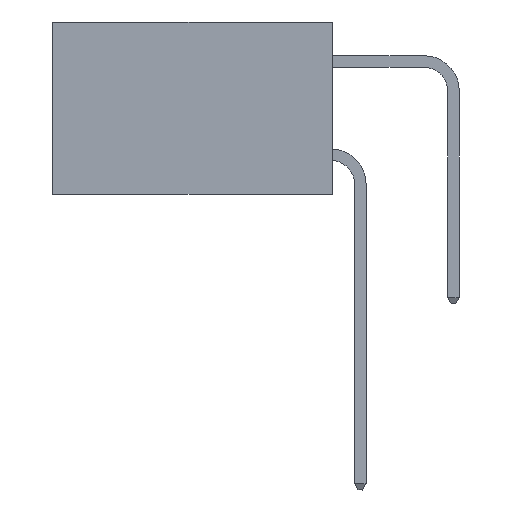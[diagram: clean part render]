
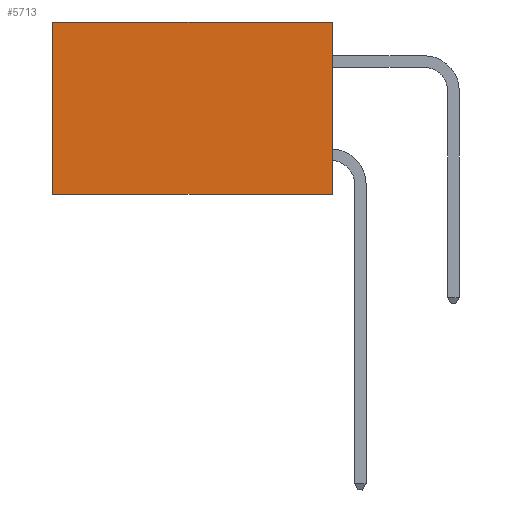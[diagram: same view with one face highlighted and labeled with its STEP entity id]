
A CAD part, left-side view. The second image highlights one B-rep face of the part: STEP entity #5713.
In plain terms, the highlighted planar face has unit normal (-1, 0, 0).
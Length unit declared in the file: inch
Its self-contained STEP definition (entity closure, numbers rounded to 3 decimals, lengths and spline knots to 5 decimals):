
#2286 = CARTESIAN_POINT ( 'NONE',  ( 0.298, 0., 0. ) ) ;
#3651 = ORIENTED_EDGE ( 'NONE', *, *, #4596, .T. ) ;
#4030 = VECTOR ( 'NONE', #24999, 39.37008 ) ;
#4124 = EDGE_CURVE ( 'NONE', #7701, #14958, #17705, .T. ) ;
#4596 = EDGE_CURVE ( 'NONE', #7062, #14991, #12025, .T. ) ;
#5713 = ADVANCED_FACE ( 'NONE', ( #29328 ), #16380, .F. ) ;
#6636 = ORIENTED_EDGE ( 'NONE', *, *, #4124, .F. ) ;
#7062 = VERTEX_POINT ( 'NONE', #23262 ) ;
#7609 = AXIS2_PLACEMENT_3D ( 'NONE', #8755, #13903, #31976 ) ;
#7701 = VERTEX_POINT ( 'NONE', #27364 ) ;
#8755 = CARTESIAN_POINT ( 'NONE',  ( 0.298, 0., 0. ) ) ;
#8858 = VECTOR ( 'NONE', #30581, 39.37008 ) ;
#10605 = CARTESIAN_POINT ( 'NONE',  ( 0.298, 0., -0.37 ) ) ;
#10717 = DIRECTION ( 'NONE',  ( 0., 1., 0. ) ) ;
#11938 = CARTESIAN_POINT ( 'NONE',  ( 0.298, 0.6, -0.37 ) ) ;
#12025 = LINE ( 'NONE', #2286, #8858 ) ;
#13350 = LINE ( 'NONE', #19286, #24247 ) ;
#13873 = ORIENTED_EDGE ( 'NONE', *, *, #21202, .F. ) ;
#13903 = DIRECTION ( 'NONE',  ( 1., 0., 0. ) ) ;
#14433 = CARTESIAN_POINT ( 'NONE',  ( 0.298, 0.6, 0. ) ) ;
#14958 = VERTEX_POINT ( 'NONE', #11938 ) ;
#14991 = VERTEX_POINT ( 'NONE', #16993 ) ;
#16380 = PLANE ( 'NONE',  #7609 ) ;
#16993 = CARTESIAN_POINT ( 'NONE',  ( 0.298, 0.6, 0. ) ) ;
#17705 = LINE ( 'NONE', #10605, #22547 ) ;
#19286 = CARTESIAN_POINT ( 'NONE',  ( 0.298, 0., 0. ) ) ;
#21202 = EDGE_CURVE ( 'NONE', #7062, #7701, #13350, .T. ) ;
#21790 = DIRECTION ( 'NONE',  ( 0., 0., -1. ) ) ;
#21914 = EDGE_CURVE ( 'NONE', #14991, #14958, #31548, .T. ) ;
#22331 = EDGE_LOOP ( 'NONE', ( #30204, #6636, #13873, #3651 ) ) ;
#22547 = VECTOR ( 'NONE', #10717, 39.37008 ) ;
#23262 = CARTESIAN_POINT ( 'NONE',  ( 0.298, 0., 0. ) ) ;
#24247 = VECTOR ( 'NONE', #21790, 39.37008 ) ;
#24999 = DIRECTION ( 'NONE',  ( 0., 0., -1. ) ) ;
#27364 = CARTESIAN_POINT ( 'NONE',  ( 0.298, 0., -0.37 ) ) ;
#29328 = FACE_OUTER_BOUND ( 'NONE', #22331, .T. ) ;
#30204 = ORIENTED_EDGE ( 'NONE', *, *, #21914, .T. ) ;
#30581 = DIRECTION ( 'NONE',  ( 0., 1., 0. ) ) ;
#31548 = LINE ( 'NONE', #14433, #4030 ) ;
#31976 = DIRECTION ( 'NONE',  ( 0., 0., -1. ) ) ;
